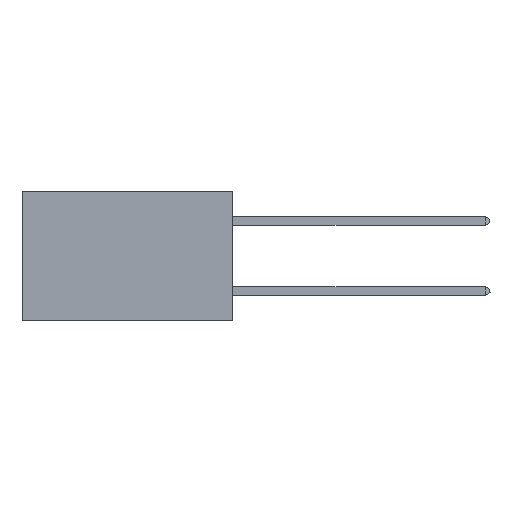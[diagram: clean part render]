
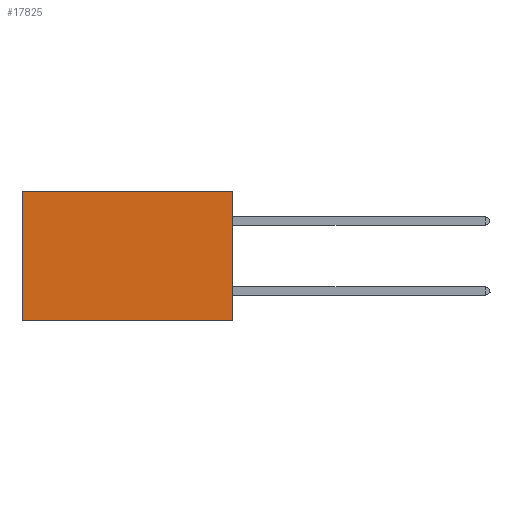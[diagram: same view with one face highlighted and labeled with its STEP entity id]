
A CAD part, left-side view. The second image highlights one B-rep face of the part: STEP entity #17825.
In plain terms, the highlighted planar face has unit normal (-1, 0, 0).
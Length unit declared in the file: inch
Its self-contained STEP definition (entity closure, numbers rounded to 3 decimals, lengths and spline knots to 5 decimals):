
#2472 = ORIENTED_EDGE ( 'NONE', *, *, #30128, .T. ) ;
#4587 = PLANE ( 'NONE',  #32104 ) ;
#5040 = CARTESIAN_POINT ( 'NONE',  ( 0.2875, 0., 0. ) ) ;
#5422 = VECTOR ( 'NONE', #9384, 39.37008 ) ;
#7578 = CARTESIAN_POINT ( 'NONE',  ( 0.2875, 0., 0. ) ) ;
#8637 = VERTEX_POINT ( 'NONE', #7578 ) ;
#9271 = VECTOR ( 'NONE', #24895, 39.37008 ) ;
#9384 = DIRECTION ( 'NONE',  ( 0., 0., -1. ) ) ;
#9411 = EDGE_CURVE ( 'NONE', #15935, #31793, #29759, .T. ) ;
#11954 = CARTESIAN_POINT ( 'NONE',  ( 0.2875, 0., 0. ) ) ;
#14167 = DIRECTION ( 'NONE',  ( 0., 1., 0. ) ) ;
#14448 = CARTESIAN_POINT ( 'NONE',  ( 0.2875, 0.6, 0. ) ) ;
#14743 = CARTESIAN_POINT ( 'NONE',  ( 0.2875, 0., 0. ) ) ;
#15246 = VERTEX_POINT ( 'NONE', #25295 ) ;
#15935 = VERTEX_POINT ( 'NONE', #28636 ) ;
#16103 = VECTOR ( 'NONE', #14167, 39.37008 ) ;
#16325 = FACE_OUTER_BOUND ( 'NONE', #17786, .T. ) ;
#16489 = CARTESIAN_POINT ( 'NONE',  ( 0.2875, 0.6, -0.37 ) ) ;
#17400 = ORIENTED_EDGE ( 'NONE', *, *, #31955, .T. ) ;
#17786 = EDGE_LOOP ( 'NONE', ( #17400, #29479, #27697, #2472 ) ) ;
#17825 = ADVANCED_FACE ( 'NONE', ( #16325 ), #4587, .F. ) ;
#18990 = CARTESIAN_POINT ( 'NONE',  ( 0.2875, 0., -0.37 ) ) ;
#19443 = LINE ( 'NONE', #14448, #27456 ) ;
#20127 = DIRECTION ( 'NONE',  ( 0., 0., -1. ) ) ;
#22900 = DIRECTION ( 'NONE',  ( 1., 0., 0. ) ) ;
#23665 = EDGE_CURVE ( 'NONE', #8637, #15935, #30698, .T. ) ;
#24895 = DIRECTION ( 'NONE',  ( 0., 1., 0. ) ) ;
#25295 = CARTESIAN_POINT ( 'NONE',  ( 0.2875, 0.6, 0. ) ) ;
#27017 = DIRECTION ( 'NONE',  ( 0., 0., -1. ) ) ;
#27456 = VECTOR ( 'NONE', #27017, 39.37008 ) ;
#27697 = ORIENTED_EDGE ( 'NONE', *, *, #23665, .F. ) ;
#28636 = CARTESIAN_POINT ( 'NONE',  ( 0.2875, 0., -0.37 ) ) ;
#29479 = ORIENTED_EDGE ( 'NONE', *, *, #9411, .F. ) ;
#29759 = LINE ( 'NONE', #18990, #16103 ) ;
#30128 = EDGE_CURVE ( 'NONE', #8637, #15246, #31345, .T. ) ;
#30698 = LINE ( 'NONE', #14743, #5422 ) ;
#31345 = LINE ( 'NONE', #11954, #9271 ) ;
#31793 = VERTEX_POINT ( 'NONE', #16489 ) ;
#31955 = EDGE_CURVE ( 'NONE', #15246, #31793, #19443, .T. ) ;
#32104 = AXIS2_PLACEMENT_3D ( 'NONE', #5040, #22900, #20127 ) ;
